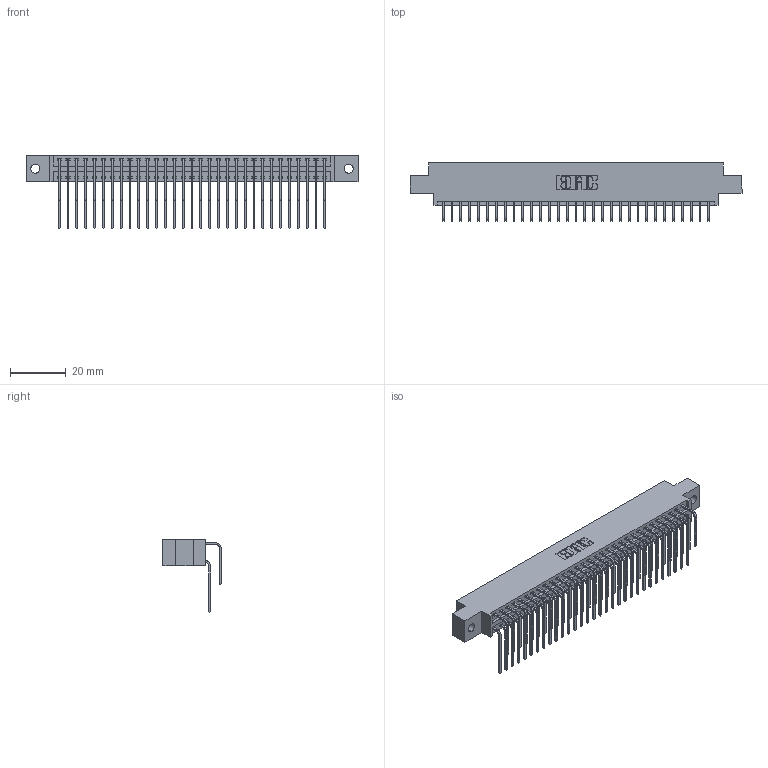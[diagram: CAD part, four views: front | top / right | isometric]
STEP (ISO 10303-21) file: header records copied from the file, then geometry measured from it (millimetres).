
FILE_DESCRIPTION (( 'STEP AP203' ), '1' );
FILE_NAME ('396-062-559-802.STEP', '2018-09-08T16:04:43', ( '' ), ( '' ), 'SwSTEP 2.0', 'SolidWorks 2016', '' );
FILE_SCHEMA (( 'CONFIG_CONTROL_DESIGN' ));
Length unit declared in the file: inch
Products named in the file (4): 346 Part_0.170 Offset - 0.128 Dia; 345-292-001_558 559 Tail - 1; 345-292-001_559 Tail - 2; 396-062-559-802
Assembly tree (63 placements, depth 2):
  396-062-559-802
    346 Part_0.170 Offset - 0.128 Dia
    345-292-001_558 559 Tail - 1  x31
    345-292-001_559 Tail - 2  x31
Bounding box: 119 x 20.89 x 26.16 mm (x, y, z)
Volume: 11684.8 mm3; surface area: 17514.9 mm2
Topology: 63 solids, 63 shells, 3474 faces, 10323 edges, 6798 vertices
Faces by surface type: plane 2374, cylinder 1100
Entity records: 23631 total; most frequent: CARTESIAN_POINT 3963, ORIENTED_EDGE 3846, DIRECTION 3515, EDGE_CURVE 1923, VECTOR 1627, LINE 1627, VERTEX_POINT 1278, AXIS2_PLACEMENT_3D 944
